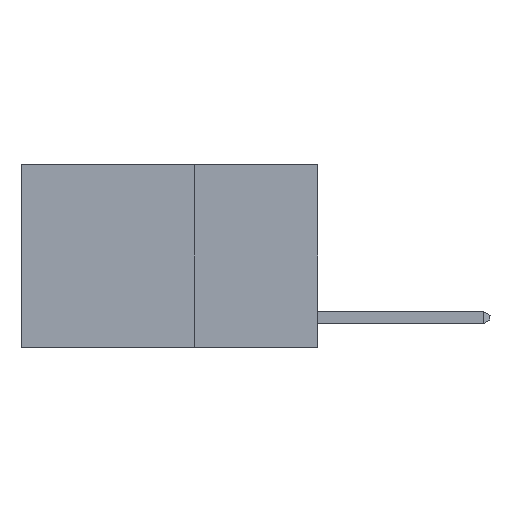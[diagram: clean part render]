
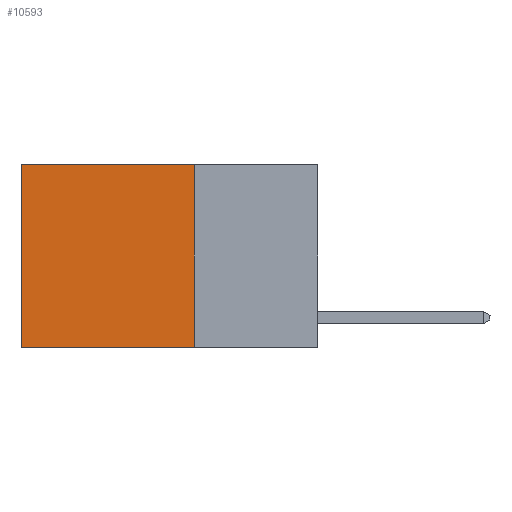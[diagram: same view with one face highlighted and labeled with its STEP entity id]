
A CAD part, left-side view. The second image highlights one B-rep face of the part: STEP entity #10593.
In plain terms, the highlighted planar face has unit normal (-1, 0, 0).
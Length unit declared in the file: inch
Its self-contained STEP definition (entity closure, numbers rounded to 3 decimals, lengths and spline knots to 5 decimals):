
#356 = CARTESIAN_POINT ( 'NONE',  ( 0.2625, 0.6, 0. ) ) ;
#515 = VERTEX_POINT ( 'NONE', #4339 ) ;
#1211 = VECTOR ( 'NONE', #1365, 39.37008 ) ;
#1365 = DIRECTION ( 'NONE',  ( 0., 0., -1. ) ) ;
#2313 = CARTESIAN_POINT ( 'NONE',  ( 0.2625, 0.6, 0. ) ) ;
#3289 = VECTOR ( 'NONE', #6090, 39.37008 ) ;
#3798 = PLANE ( 'NONE',  #8339 ) ;
#4308 = EDGE_CURVE ( 'NONE', #10103, #11951, #10157, .T. ) ;
#4339 = CARTESIAN_POINT ( 'NONE',  ( 0.2625, 0.25, 0. ) ) ;
#4351 = ORIENTED_EDGE ( 'NONE', *, *, #8813, .T. ) ;
#4424 = EDGE_CURVE ( 'NONE', #515, #10103, #8958, .T. ) ;
#4574 = ORIENTED_EDGE ( 'NONE', *, *, #11627, .T. ) ;
#4829 = DIRECTION ( 'NONE',  ( 1., 0., 0. ) ) ;
#5555 = CARTESIAN_POINT ( 'NONE',  ( 0.2625, 0.6, -0.37 ) ) ;
#5797 = VERTEX_POINT ( 'NONE', #2313 ) ;
#5897 = ORIENTED_EDGE ( 'NONE', *, *, #4424, .F. ) ;
#5959 = DIRECTION ( 'NONE',  ( 0., 0., -1. ) ) ;
#5963 = LINE ( 'NONE', #11689, #3289 ) ;
#6090 = DIRECTION ( 'NONE',  ( 0., 1., 0. ) ) ;
#6753 = DIRECTION ( 'NONE',  ( 0., 1., 0. ) ) ;
#7016 = EDGE_LOOP ( 'NONE', ( #4351, #10905, #5897, #4574 ) ) ;
#7468 = FACE_OUTER_BOUND ( 'NONE', #7016, .T. ) ;
#8339 = AXIS2_PLACEMENT_3D ( 'NONE', #10636, #4829, #11618 ) ;
#8457 = CARTESIAN_POINT ( 'NONE',  ( 0.2625, 0.25, -0.37 ) ) ;
#8644 = VECTOR ( 'NONE', #5959, 39.37008 ) ;
#8813 = EDGE_CURVE ( 'NONE', #5797, #11951, #9038, .T. ) ;
#8958 = LINE ( 'NONE', #10742, #8644 ) ;
#9038 = LINE ( 'NONE', #356, #1211 ) ;
#10103 = VERTEX_POINT ( 'NONE', #8457 ) ;
#10157 = LINE ( 'NONE', #10567, #12427 ) ;
#10567 = CARTESIAN_POINT ( 'NONE',  ( 0.2625, 0.25, -0.37 ) ) ;
#10593 = ADVANCED_FACE ( 'NONE', ( #7468 ), #3798, .F. ) ;
#10636 = CARTESIAN_POINT ( 'NONE',  ( 0.2625, 0.25, 0. ) ) ;
#10742 = CARTESIAN_POINT ( 'NONE',  ( 0.2625, 0.25, 0. ) ) ;
#10905 = ORIENTED_EDGE ( 'NONE', *, *, #4308, .F. ) ;
#11618 = DIRECTION ( 'NONE',  ( 0., 0., -1. ) ) ;
#11627 = EDGE_CURVE ( 'NONE', #515, #5797, #5963, .T. ) ;
#11689 = CARTESIAN_POINT ( 'NONE',  ( 0.2625, 0.25, 0. ) ) ;
#11951 = VERTEX_POINT ( 'NONE', #5555 ) ;
#12427 = VECTOR ( 'NONE', #6753, 39.37008 ) ;
